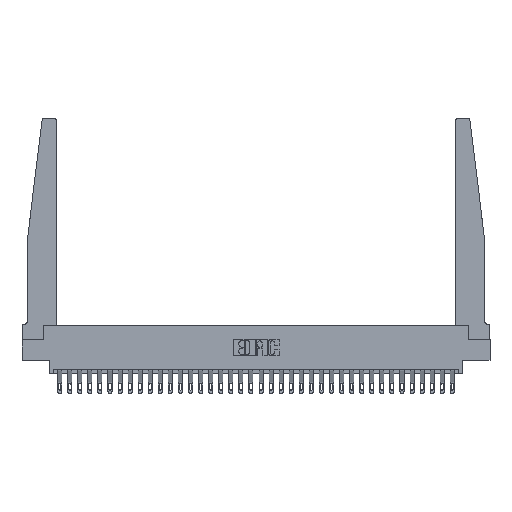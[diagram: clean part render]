
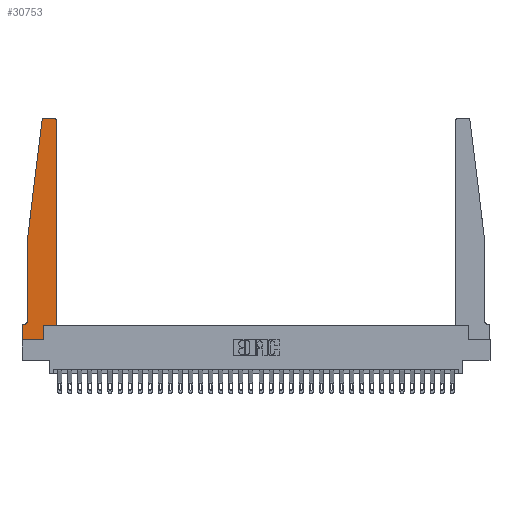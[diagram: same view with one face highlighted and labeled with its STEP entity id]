
A CAD part, top view. The second image highlights one B-rep face of the part: STEP entity #30753.
In plain terms, the highlighted planar face has unit normal (0, 0, 1).
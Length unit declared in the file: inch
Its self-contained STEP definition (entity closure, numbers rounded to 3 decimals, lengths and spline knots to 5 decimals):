
#4 = ORIENTED_EDGE ( 'NONE', *, *, #23885, .T. ) ;
#159 = VERTEX_POINT ( 'NONE', #19382 ) ;
#187 = ORIENTED_EDGE ( 'NONE', *, *, #29463, .T. ) ;
#608 = AXIS2_PLACEMENT_3D ( 'NONE', #5618, #22711, #8044 ) ;
#709 = VECTOR ( 'NONE', #31316, 39.37008 ) ;
#938 = CARTESIAN_POINT ( 'NONE',  ( 0.395, 2.72, 0.37 ) ) ;
#1013 = VERTEX_POINT ( 'NONE', #22193 ) ;
#1240 = DIRECTION ( 'NONE',  ( 1., 0., 0. ) ) ;
#1638 = VERTEX_POINT ( 'NONE', #26757 ) ;
#1807 = CARTESIAN_POINT ( 'NONE',  ( 0.425, 0.18, 0.37 ) ) ;
#2021 = VECTOR ( 'NONE', #30820, 39.37008 ) ;
#3043 = VERTEX_POINT ( 'NONE', #8484 ) ;
#3191 = DIRECTION ( 'NONE',  ( 0., -1., 0. ) ) ;
#3216 = ORIENTED_EDGE ( 'NONE', *, *, #8729, .T. ) ;
#3246 = CARTESIAN_POINT ( 'NONE',  ( 0., 0., 0.37 ) ) ;
#3362 = DIRECTION ( 'NONE',  ( 1., 0., 0. ) ) ;
#3795 = CARTESIAN_POINT ( 'NONE',  ( 0.24675, 2.72367, 0.37 ) ) ;
#4523 = CARTESIAN_POINT ( 'NONE',  ( 0.2605, 0., 0.37 ) ) ;
#4542 = LINE ( 'NONE', #13027, #30537 ) ;
#4596 = CARTESIAN_POINT ( 'NONE',  ( 0.065, 1.25, 0.37 ) ) ;
#5262 = VECTOR ( 'NONE', #15444, 39.37008 ) ;
#5466 = EDGE_CURVE ( 'NONE', #9576, #17127, #10988, .T. ) ;
#5495 = DIRECTION ( 'NONE',  ( 0., -1., 0. ) ) ;
#5516 = AXIS2_PLACEMENT_3D ( 'NONE', #938, #18023, #3362 ) ;
#5618 = CARTESIAN_POINT ( 'NONE',  ( 0.015, 0.2375, 0.37 ) ) ;
#5695 = DIRECTION ( 'NONE',  ( 1., 0., 0. ) ) ;
#6097 = ORIENTED_EDGE ( 'NONE', *, *, #14623, .T. ) ;
#6762 = AXIS2_PLACEMENT_3D ( 'NONE', #29263, #14629, #1240 ) ;
#6809 = FACE_OUTER_BOUND ( 'NONE', #30407, .T. ) ;
#8044 = DIRECTION ( 'NONE',  ( -1., 0., 0. ) ) ;
#8087 = CIRCLE ( 'NONE', #6762, 0.03 ) ;
#8290 = VERTEX_POINT ( 'NONE', #19440 ) ;
#8463 = VECTOR ( 'NONE', #12698, 39.37008 ) ;
#8484 = CARTESIAN_POINT ( 'NONE',  ( 0.2605, 0.18, 0.37 ) ) ;
#8729 = EDGE_CURVE ( 'NONE', #13744, #9576, #8087, .T. ) ;
#9576 = VERTEX_POINT ( 'NONE', #3795 ) ;
#9865 = VECTOR ( 'NONE', #5695, 39.37008 ) ;
#10321 = LINE ( 'NONE', #1807, #22547 ) ;
#10346 = DIRECTION ( 'NONE',  ( 1., 0., 0. ) ) ;
#10988 = LINE ( 'NONE', #12990, #5262 ) ;
#10994 = EDGE_CURVE ( 'NONE', #1013, #13744, #15025, .T. ) ;
#11495 = ORIENTED_EDGE ( 'NONE', *, *, #10994, .T. ) ;
#11834 = EDGE_CURVE ( 'NONE', #8290, #29865, #25325, .T. ) ;
#12698 = DIRECTION ( 'NONE',  ( 1., 0., 0. ) ) ;
#12990 = CARTESIAN_POINT ( 'NONE',  ( 0.065, 1.25, 0.37 ) ) ;
#13027 = CARTESIAN_POINT ( 'NONE',  ( 0.065, 1.25, 0.37 ) ) ;
#13744 = VERTEX_POINT ( 'NONE', #29849 ) ;
#14623 = EDGE_CURVE ( 'NONE', #159, #8290, #20218, .T. ) ;
#14626 = VECTOR ( 'NONE', #5495, 39.37008 ) ;
#14629 = DIRECTION ( 'NONE',  ( 0., 0., 1. ) ) ;
#14873 = CIRCLE ( 'NONE', #608, 0.05 ) ;
#15025 = LINE ( 'NONE', #23465, #2021 ) ;
#15079 = VERTEX_POINT ( 'NONE', #4523 ) ;
#15444 = DIRECTION ( 'NONE',  ( -0.122, -0.992, 0. ) ) ;
#15480 = EDGE_CURVE ( 'NONE', #15079, #3043, #23172, .T. ) ;
#16119 = ORIENTED_EDGE ( 'NONE', *, *, #27460, .T. ) ;
#16538 = CARTESIAN_POINT ( 'NONE',  ( 0.425, 0.18, 0.37 ) ) ;
#16688 = CARTESIAN_POINT ( 'NONE',  ( 0.065, 0.1875, 0.37 ) ) ;
#17127 = VERTEX_POINT ( 'NONE', #4596 ) ;
#17132 = LINE ( 'NONE', #3246, #9865 ) ;
#18023 = DIRECTION ( 'NONE',  ( 0., 0., 1. ) ) ;
#18255 = ORIENTED_EDGE ( 'NONE', *, *, #29423, .T. ) ;
#18907 = DIRECTION ( 'NONE',  ( 0., 1., 0. ) ) ;
#19382 = CARTESIAN_POINT ( 'NONE',  ( 0.015, 0.1875, 0.37 ) ) ;
#19440 = CARTESIAN_POINT ( 'NONE',  ( 0., 0.1875, 0.37 ) ) ;
#19867 = CIRCLE ( 'NONE', #5516, 0.03 ) ;
#20096 = PLANE ( 'NONE',  #26595 ) ;
#20218 = LINE ( 'NONE', #16688, #709 ) ;
#21450 = EDGE_CURVE ( 'NONE', #26336, #29460, #10321, .T. ) ;
#21492 = LINE ( 'NONE', #29783, #8463 ) ;
#21818 = CARTESIAN_POINT ( 'NONE',  ( 0., 0., 0.37 ) ) ;
#22193 = CARTESIAN_POINT ( 'NONE',  ( 0.395, 2.75, 0.37 ) ) ;
#22410 = VECTOR ( 'NONE', #27010, 39.37008 ) ;
#22522 = CARTESIAN_POINT ( 'NONE',  ( 0., 0.1875, 0.37 ) ) ;
#22547 = VECTOR ( 'NONE', #18907, 39.37008 ) ;
#22711 = DIRECTION ( 'NONE',  ( 0., 0., -1. ) ) ;
#22809 = CARTESIAN_POINT ( 'NONE',  ( 0.425, 2.72, 0.37 ) ) ;
#23172 = LINE ( 'NONE', #29376, #22410 ) ;
#23465 = CARTESIAN_POINT ( 'NONE',  ( 0.25, 2.75, 0.37 ) ) ;
#23885 = EDGE_CURVE ( 'NONE', #29865, #15079, #17132, .T. ) ;
#24987 = DIRECTION ( 'NONE',  ( 0., 0., 1. ) ) ;
#25325 = LINE ( 'NONE', #29955, #14626 ) ;
#25592 = ORIENTED_EDGE ( 'NONE', *, *, #15480, .T. ) ;
#26336 = VERTEX_POINT ( 'NONE', #16538 ) ;
#26595 = AXIS2_PLACEMENT_3D ( 'NONE', #22522, #24987, #10346 ) ;
#26757 = CARTESIAN_POINT ( 'NONE',  ( 0.065, 0.2375, 0.37 ) ) ;
#27010 = DIRECTION ( 'NONE',  ( 0., 1., 0. ) ) ;
#27030 = ORIENTED_EDGE ( 'NONE', *, *, #30830, .T. ) ;
#27460 = EDGE_CURVE ( 'NONE', #3043, #26336, #21492, .T. ) ;
#28778 = ORIENTED_EDGE ( 'NONE', *, *, #5466, .T. ) ;
#29263 = CARTESIAN_POINT ( 'NONE',  ( 0.27653, 2.72, 0.37 ) ) ;
#29376 = CARTESIAN_POINT ( 'NONE',  ( 0.2605, 0.18, 0.37 ) ) ;
#29423 = EDGE_CURVE ( 'NONE', #1638, #159, #14873, .T. ) ;
#29460 = VERTEX_POINT ( 'NONE', #22809 ) ;
#29463 = EDGE_CURVE ( 'NONE', #29460, #1013, #19867, .T. ) ;
#29783 = CARTESIAN_POINT ( 'NONE',  ( 0.425, 0.18, 0.37 ) ) ;
#29801 = ORIENTED_EDGE ( 'NONE', *, *, #21450, .T. ) ;
#29849 = CARTESIAN_POINT ( 'NONE',  ( 0.27653, 2.75, 0.37 ) ) ;
#29865 = VERTEX_POINT ( 'NONE', #21818 ) ;
#29955 = CARTESIAN_POINT ( 'NONE',  ( 0., 0., 0.37 ) ) ;
#30407 = EDGE_LOOP ( 'NONE', ( #11495, #3216, #28778, #27030, #18255, #6097, #30585, #4, #25592, #16119, #29801, #187 ) ) ;
#30537 = VECTOR ( 'NONE', #3191, 39.37008 ) ;
#30585 = ORIENTED_EDGE ( 'NONE', *, *, #11834, .T. ) ;
#30753 = ADVANCED_FACE ( 'NONE', ( #6809 ), #20096, .T. ) ;
#30820 = DIRECTION ( 'NONE',  ( -1., 0., 0. ) ) ;
#30830 = EDGE_CURVE ( 'NONE', #17127, #1638, #4542, .T. ) ;
#31316 = DIRECTION ( 'NONE',  ( -1., 0., 0. ) ) ;
